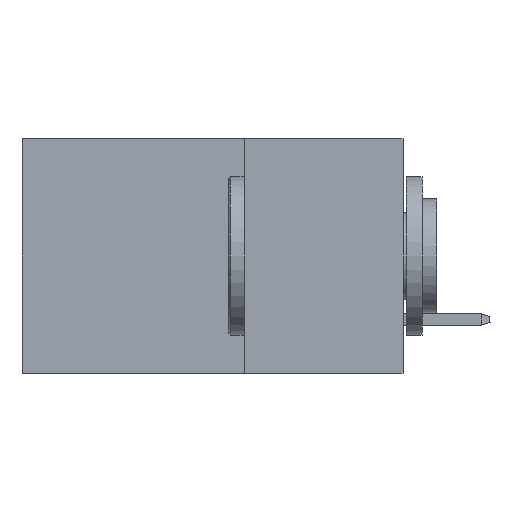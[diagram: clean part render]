
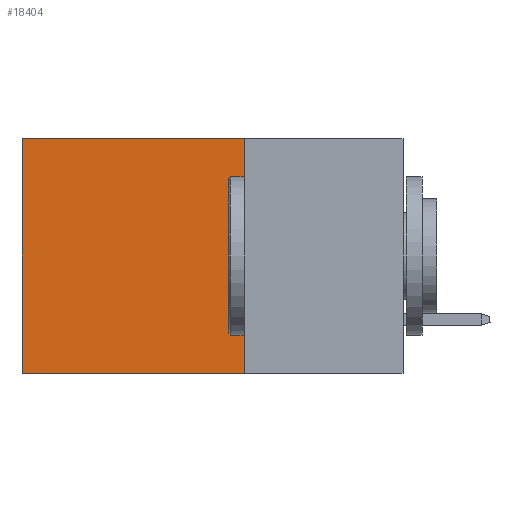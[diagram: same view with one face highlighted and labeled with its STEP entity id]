
A CAD part, left-side view. The second image highlights one B-rep face of the part: STEP entity #18404.
In plain terms, the highlighted planar face has unit normal (-1, 0, 0).
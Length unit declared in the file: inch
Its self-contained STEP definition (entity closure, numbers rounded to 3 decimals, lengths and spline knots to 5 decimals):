
#100 = CARTESIAN_POINT ( 'NONE',  ( 0.2875, 0.25, 0. ) ) ;
#512 = EDGE_CURVE ( 'NONE', #7877, #3998, #18083, .T. ) ;
#1238 = DIRECTION ( 'NONE',  ( 0., 0., -1. ) ) ;
#1362 = VECTOR ( 'NONE', #3233, 39.37008 ) ;
#2322 = EDGE_LOOP ( 'NONE', ( #4025, #12933, #15110, #8360 ) ) ;
#3116 = CARTESIAN_POINT ( 'NONE',  ( 0.2875, 0.25, 0. ) ) ;
#3233 = DIRECTION ( 'NONE',  ( 0., 0., -1. ) ) ;
#3478 = VERTEX_POINT ( 'NONE', #21906 ) ;
#3998 = VERTEX_POINT ( 'NONE', #8736 ) ;
#4025 = ORIENTED_EDGE ( 'NONE', *, *, #512, .T. ) ;
#4839 = LINE ( 'NONE', #17739, #9469 ) ;
#4943 = DIRECTION ( 'NONE',  ( 0., 0., -1. ) ) ;
#7028 = CARTESIAN_POINT ( 'NONE',  ( 0.2875, 0.6, 0. ) ) ;
#7595 = DIRECTION ( 'NONE',  ( 1., 0., 0. ) ) ;
#7877 = VERTEX_POINT ( 'NONE', #20707 ) ;
#8289 = EDGE_CURVE ( 'NONE', #3478, #7877, #4839, .T. ) ;
#8360 = ORIENTED_EDGE ( 'NONE', *, *, #8289, .T. ) ;
#8736 = CARTESIAN_POINT ( 'NONE',  ( 0.2875, 0.6, -0.37 ) ) ;
#9469 = VECTOR ( 'NONE', #19709, 39.37008 ) ;
#11940 = VECTOR ( 'NONE', #13136, 39.37008 ) ;
#12933 = ORIENTED_EDGE ( 'NONE', *, *, #20141, .F. ) ;
#13136 = DIRECTION ( 'NONE',  ( 0., 1., 0. ) ) ;
#13404 = EDGE_CURVE ( 'NONE', #3478, #18463, #20069, .T. ) ;
#14264 = PLANE ( 'NONE',  #22703 ) ;
#15107 = LINE ( 'NONE', #18546, #11940 ) ;
#15110 = ORIENTED_EDGE ( 'NONE', *, *, #13404, .F. ) ;
#16947 = FACE_OUTER_BOUND ( 'NONE', #2322, .T. ) ;
#17739 = CARTESIAN_POINT ( 'NONE',  ( 0.2875, 0.25, 0. ) ) ;
#18083 = LINE ( 'NONE', #7028, #21488 ) ;
#18404 = ADVANCED_FACE ( 'NONE', ( #16947 ), #14264, .F. ) ;
#18463 = VERTEX_POINT ( 'NONE', #19010 ) ;
#18546 = CARTESIAN_POINT ( 'NONE',  ( 0.2875, 0.25, -0.37 ) ) ;
#19010 = CARTESIAN_POINT ( 'NONE',  ( 0.2875, 0.25, -0.37 ) ) ;
#19709 = DIRECTION ( 'NONE',  ( 0., 1., 0. ) ) ;
#20069 = LINE ( 'NONE', #3116, #1362 ) ;
#20141 = EDGE_CURVE ( 'NONE', #18463, #3998, #15107, .T. ) ;
#20707 = CARTESIAN_POINT ( 'NONE',  ( 0.2875, 0.6, 0. ) ) ;
#21488 = VECTOR ( 'NONE', #4943, 39.37008 ) ;
#21906 = CARTESIAN_POINT ( 'NONE',  ( 0.2875, 0.25, 0. ) ) ;
#22703 = AXIS2_PLACEMENT_3D ( 'NONE', #100, #7595, #1238 ) ;
